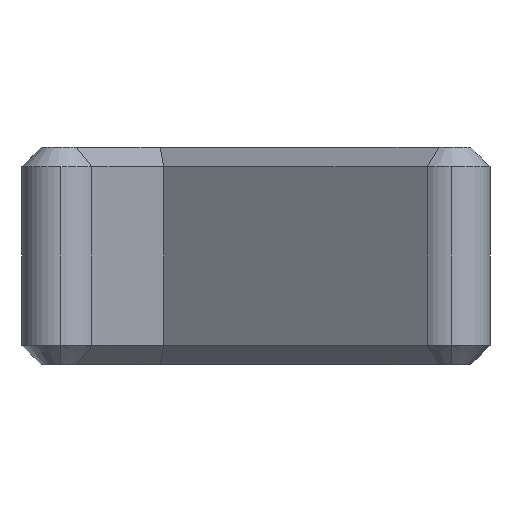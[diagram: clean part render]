
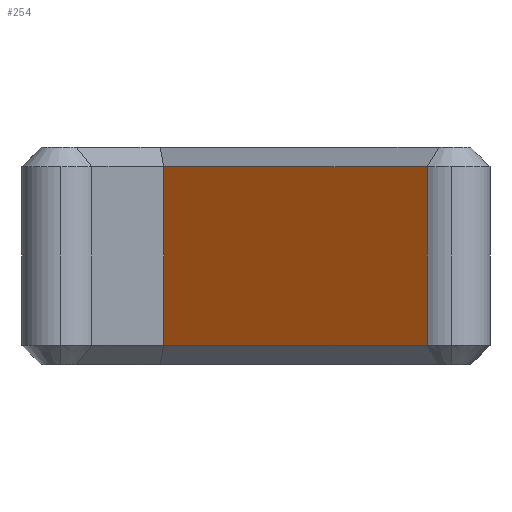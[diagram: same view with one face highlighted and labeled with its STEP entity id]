
A CAD part, front view. The second image highlights one B-rep face of the part: STEP entity #254.
In plain terms, the highlighted planar face has unit normal (-0.613, -0.79, 0).
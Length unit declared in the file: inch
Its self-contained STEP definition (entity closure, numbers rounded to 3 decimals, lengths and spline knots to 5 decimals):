
#13 = CARTESIAN_POINT ( 'NONE',  ( 0.352, -0.48261, 0.06252 ) ) ;
#235 = LINE ( 'NONE', #899, #1083 ) ;
#241 = ORIENTED_EDGE ( 'NONE', *, *, #724, .T. ) ;
#251 = EDGE_CURVE ( 'NONE', #436, #279, #1707, .T. ) ;
#254 = ADVANCED_FACE ( 'NONE', ( #959 ), #497, .F. ) ;
#267 = CARTESIAN_POINT ( 'NONE',  ( -0.15438, -0.08998, -0.28079 ) ) ;
#279 = VERTEX_POINT ( 'NONE', #361 ) ;
#361 = CARTESIAN_POINT ( 'NONE',  ( -0.15438, -0.08998, 0.06252 ) ) ;
#385 = DIRECTION ( 'NONE',  ( 0.79, -0.613, 0. ) ) ;
#436 = VERTEX_POINT ( 'NONE', #267 ) ;
#497 = PLANE ( 'NONE',  #562 ) ;
#501 = DIRECTION ( 'NONE',  ( 0.613, 0.79, 0. ) ) ;
#509 = DIRECTION ( 'NONE',  ( 0., 0., 1. ) ) ;
#515 = ORIENTED_EDGE ( 'NONE', *, *, #251, .F. ) ;
#562 = AXIS2_PLACEMENT_3D ( 'NONE', #1545, #501, #636 ) ;
#618 = VECTOR ( 'NONE', #385, 39.37008 ) ;
#632 = CARTESIAN_POINT ( 'NONE',  ( -0.15438, -0.08998, -0.31829 ) ) ;
#636 = DIRECTION ( 'NONE',  ( 0.79, -0.613, 0. ) ) ;
#650 = DIRECTION ( 'NONE',  ( 0., 0., 1. ) ) ;
#724 = EDGE_CURVE ( 'NONE', #1028, #279, #777, .T. ) ;
#754 = EDGE_CURVE ( 'NONE', #848, #1028, #235, .T. ) ;
#764 = ORIENTED_EDGE ( 'NONE', *, *, #754, .T. ) ;
#777 = LINE ( 'NONE', #1548, #1146 ) ;
#808 = EDGE_LOOP ( 'NONE', ( #515, #926, #764, #241 ) ) ;
#827 = EDGE_CURVE ( 'NONE', #436, #848, #1124, .T. ) ;
#848 = VERTEX_POINT ( 'NONE', #1702 ) ;
#899 = CARTESIAN_POINT ( 'NONE',  ( 0.352, -0.48261, -0.31829 ) ) ;
#907 = DIRECTION ( 'NONE',  ( -0.79, 0.613, 0. ) ) ;
#926 = ORIENTED_EDGE ( 'NONE', *, *, #827, .T. ) ;
#959 = FACE_OUTER_BOUND ( 'NONE', #808, .T. ) ;
#1028 = VERTEX_POINT ( 'NONE', #13 ) ;
#1083 = VECTOR ( 'NONE', #509, 39.37008 ) ;
#1124 = LINE ( 'NONE', #1587, #618 ) ;
#1146 = VECTOR ( 'NONE', #907, 39.37008 ) ;
#1308 = VECTOR ( 'NONE', #650, 39.37008 ) ;
#1545 = CARTESIAN_POINT ( 'NONE',  ( -0.15438, -0.08998, -0.31829 ) ) ;
#1548 = CARTESIAN_POINT ( 'NONE',  ( -0.15438, -0.08998, 0.06252 ) ) ;
#1587 = CARTESIAN_POINT ( 'NONE',  ( -0.15438, -0.08998, -0.28079 ) ) ;
#1702 = CARTESIAN_POINT ( 'NONE',  ( 0.352, -0.48261, -0.28079 ) ) ;
#1707 = LINE ( 'NONE', #632, #1308 ) ;
